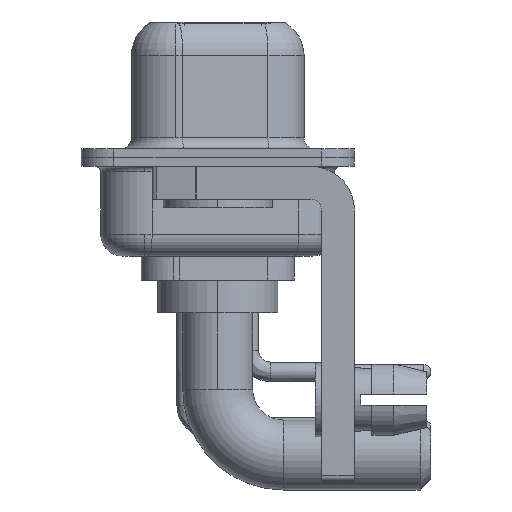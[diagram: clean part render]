
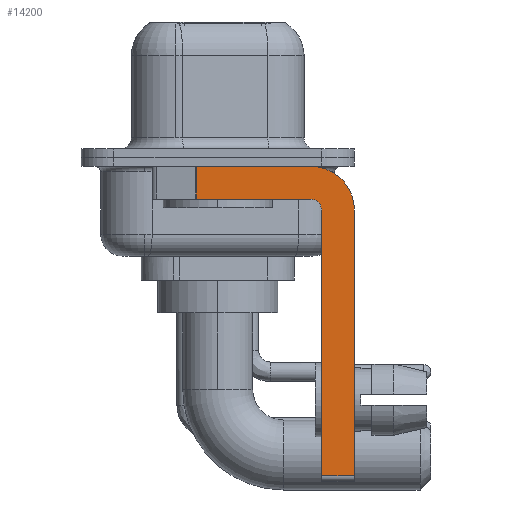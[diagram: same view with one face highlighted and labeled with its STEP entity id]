
A CAD part, left-side view. The second image highlights one B-rep face of the part: STEP entity #14200.
In plain terms, the highlighted planar face has unit normal (-1, 0, 0).
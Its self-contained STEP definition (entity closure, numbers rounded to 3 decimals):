
#214 = DIRECTION ( 'NONE',  ( 1., 0., 0. ) ) ;
#251 = VERTEX_POINT ( 'NONE', #13316 ) ;
#406 = CARTESIAN_POINT ( 'NONE',  ( -2.9, -4.25, -2.4 ) ) ;
#485 = CARTESIAN_POINT ( 'NONE',  ( -2.9, 0.978, -1.9 ) ) ;
#509 = ORIENTED_EDGE ( 'NONE', *, *, #17925, .F. ) ;
#969 = DIRECTION ( 'NONE',  ( 0., 0., -1. ) ) ;
#1877 = DIRECTION ( 'NONE',  ( 0., -1., 0. ) ) ;
#2091 = EDGE_CURVE ( 'NONE', #15694, #16707, #2221, .T. ) ;
#2221 = LINE ( 'NONE', #8359, #3486 ) ;
#2308 = VECTOR ( 'NONE', #16363, 1000. ) ;
#2513 = VERTEX_POINT ( 'NONE', #11443 ) ;
#2887 = CARTESIAN_POINT ( 'NONE',  ( -2.9, -6.25, -2.4 ) ) ;
#2947 = VECTOR ( 'NONE', #15630, 1000. ) ;
#3039 = PLANE ( 'NONE',  #16531 ) ;
#3253 = VECTOR ( 'NONE', #969, 1000. ) ;
#3486 = VECTOR ( 'NONE', #6790, 1000. ) ;
#3604 = VERTEX_POINT ( 'NONE', #10422 ) ;
#3753 = ORIENTED_EDGE ( 'NONE', *, *, #16121, .T. ) ;
#3766 = ORIENTED_EDGE ( 'NONE', *, *, #4598, .F. ) ;
#4302 = CARTESIAN_POINT ( 'NONE',  ( -2.9, -4.75, -2.4 ) ) ;
#4583 = CARTESIAN_POINT ( 'NONE',  ( -2.9, -4.25, -2.4 ) ) ;
#4598 = EDGE_CURVE ( 'NONE', #3604, #18460, #8482, .T. ) ;
#4806 = CARTESIAN_POINT ( 'NONE',  ( -2.9, -4.25, -14.55 ) ) ;
#4892 = LINE ( 'NONE', #4806, #11351 ) ;
#5320 = CIRCLE ( 'NONE', #15285, 2. ) ;
#5552 = DIRECTION ( 'NONE',  ( 0., 0., 1. ) ) ;
#5666 = CARTESIAN_POINT ( 'NONE',  ( -2.9, 0.978, -0.4 ) ) ;
#5819 = CARTESIAN_POINT ( 'NONE',  ( -2.9, 0.978, -1.9 ) ) ;
#6396 = VERTEX_POINT ( 'NONE', #2887 ) ;
#6549 = CIRCLE ( 'NONE', #13095, 0.5 ) ;
#6790 = DIRECTION ( 'NONE',  ( 0., 0., 1. ) ) ;
#7682 = ORIENTED_EDGE ( 'NONE', *, *, #2091, .F. ) ;
#7925 = DIRECTION ( 'NONE',  ( 0., 0., -1. ) ) ;
#8359 = CARTESIAN_POINT ( 'NONE',  ( -2.9, -4.75, -14.8 ) ) ;
#8482 = LINE ( 'NONE', #18974, #10020 ) ;
#8606 = CARTESIAN_POINT ( 'NONE',  ( -2.9, -4.25, -2.4 ) ) ;
#10008 = ORIENTED_EDGE ( 'NONE', *, *, #10330, .T. ) ;
#10020 = VECTOR ( 'NONE', #19087, 1000. ) ;
#10330 = EDGE_CURVE ( 'NONE', #15694, #251, #4892, .T. ) ;
#10422 = CARTESIAN_POINT ( 'NONE',  ( -2.9, -4.25, -1.9 ) ) ;
#11022 = EDGE_CURVE ( 'NONE', #6396, #251, #18605, .T. ) ;
#11058 = ORIENTED_EDGE ( 'NONE', *, *, #16684, .F. ) ;
#11351 = VECTOR ( 'NONE', #1877, 1000. ) ;
#11424 = CARTESIAN_POINT ( 'NONE',  ( -2.9, -6.25, -2.4 ) ) ;
#11443 = CARTESIAN_POINT ( 'NONE',  ( -2.9, -4.25, -0.4 ) ) ;
#11627 = EDGE_LOOP ( 'NONE', ( #11058, #3753, #3766, #509, #7682, #10008, #18091, #18119 ) ) ;
#12103 = FACE_OUTER_BOUND ( 'NONE', #11627, .T. ) ;
#13095 = AXIS2_PLACEMENT_3D ( 'NONE', #8606, #15894, #5552 ) ;
#13316 = CARTESIAN_POINT ( 'NONE',  ( -2.9, -6.25, -14.55 ) ) ;
#13752 = DIRECTION ( 'NONE',  ( 0., 0., -1. ) ) ;
#13858 = DIRECTION ( 'NONE',  ( 1., 0., 0. ) ) ;
#14069 = CARTESIAN_POINT ( 'NONE',  ( -2.9, 3., -0.4 ) ) ;
#14200 = ADVANCED_FACE ( 'NONE', ( #12103 ), #3039, .F. ) ;
#14225 = EDGE_CURVE ( 'NONE', #2513, #6396, #5320, .T. ) ;
#15283 = LINE ( 'NONE', #485, #2308 ) ;
#15285 = AXIS2_PLACEMENT_3D ( 'NONE', #406, #214, #7925 ) ;
#15630 = DIRECTION ( 'NONE',  ( 0., -1., 0. ) ) ;
#15694 = VERTEX_POINT ( 'NONE', #15791 ) ;
#15791 = CARTESIAN_POINT ( 'NONE',  ( -2.9, -4.75, -14.55 ) ) ;
#15894 = DIRECTION ( 'NONE',  ( -1., 0., 0. ) ) ;
#16121 = EDGE_CURVE ( 'NONE', #19086, #18460, #15283, .T. ) ;
#16363 = DIRECTION ( 'NONE',  ( 0., 0., -1. ) ) ;
#16531 = AXIS2_PLACEMENT_3D ( 'NONE', #4583, #13858, #13752 ) ;
#16684 = EDGE_CURVE ( 'NONE', #19086, #2513, #17464, .T. ) ;
#16707 = VERTEX_POINT ( 'NONE', #4302 ) ;
#17464 = LINE ( 'NONE', #14069, #2947 ) ;
#17925 = EDGE_CURVE ( 'NONE', #16707, #3604, #6549, .T. ) ;
#18091 = ORIENTED_EDGE ( 'NONE', *, *, #11022, .F. ) ;
#18119 = ORIENTED_EDGE ( 'NONE', *, *, #14225, .F. ) ;
#18460 = VERTEX_POINT ( 'NONE', #5819 ) ;
#18605 = LINE ( 'NONE', #11424, #3253 ) ;
#18974 = CARTESIAN_POINT ( 'NONE',  ( -2.9, -4.25, -1.9 ) ) ;
#19086 = VERTEX_POINT ( 'NONE', #5666 ) ;
#19087 = DIRECTION ( 'NONE',  ( 0., 1., 0. ) ) ;
